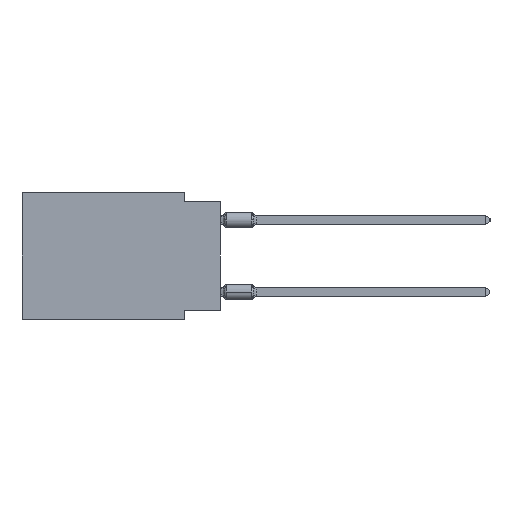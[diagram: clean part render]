
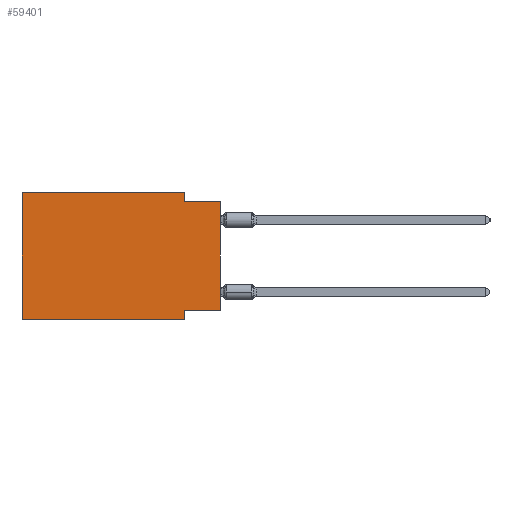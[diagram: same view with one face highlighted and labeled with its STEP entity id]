
A CAD part, left-side view. The second image highlights one B-rep face of the part: STEP entity #59401.
In plain terms, the highlighted planar face has unit normal (-1, 0, 0).
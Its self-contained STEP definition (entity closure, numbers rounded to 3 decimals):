
#155 = ORIENTED_EDGE ( 'NONE', *, *, #10946, .F. ) ;
#439 = DIRECTION ( 'NONE',  ( 0., -1., 0. ) ) ;
#2168 = DIRECTION ( 'NONE',  ( 0., 0., -1. ) ) ;
#2328 = CARTESIAN_POINT ( 'NONE',  ( 0., 13.97, -8.89 ) ) ;
#3798 = CARTESIAN_POINT ( 'NONE',  ( 0., 13.97, 0. ) ) ;
#4429 = DIRECTION ( 'NONE',  ( 0., 0., 1. ) ) ;
#4997 = VERTEX_POINT ( 'NONE', #58308 ) ;
#5055 = LINE ( 'NONE', #38365, #21850 ) ;
#5724 = VERTEX_POINT ( 'NONE', #56648 ) ;
#5874 = VECTOR ( 'NONE', #4429, 1000. ) ;
#6371 = CARTESIAN_POINT ( 'NONE',  ( 0., 0., -8.255 ) ) ;
#6458 = CARTESIAN_POINT ( 'NONE',  ( 0., 2.54, -8.89 ) ) ;
#7206 = VECTOR ( 'NONE', #55084, 1000. ) ;
#7301 = EDGE_CURVE ( 'NONE', #29168, #5724, #11497, .T. ) ;
#7315 = DIRECTION ( 'NONE',  ( 0., -1., 0. ) ) ;
#7899 = CARTESIAN_POINT ( 'NONE',  ( 0., 13.97, -8.89 ) ) ;
#8772 = VECTOR ( 'NONE', #9149, 1000. ) ;
#8821 = LINE ( 'NONE', #27630, #56164 ) ;
#9149 = DIRECTION ( 'NONE',  ( 0., 1., 0. ) ) ;
#9258 = VERTEX_POINT ( 'NONE', #46774 ) ;
#9321 = EDGE_CURVE ( 'NONE', #30063, #37108, #8821, .T. ) ;
#9517 = ORIENTED_EDGE ( 'NONE', *, *, #58188, .F. ) ;
#9600 = EDGE_LOOP ( 'NONE', ( #11555, #54944, #9517, #24430, #43706, #43105, #25051, #155 ) ) ;
#9776 = VECTOR ( 'NONE', #7315, 1000. ) ;
#10946 = EDGE_CURVE ( 'NONE', #29168, #9258, #13748, .T. ) ;
#11497 = LINE ( 'NONE', #24757, #60347 ) ;
#11555 = ORIENTED_EDGE ( 'NONE', *, *, #7301, .T. ) ;
#13257 = VERTEX_POINT ( 'NONE', #2328 ) ;
#13748 = LINE ( 'NONE', #51395, #8772 ) ;
#14059 = AXIS2_PLACEMENT_3D ( 'NONE', #25601, #31442, #2168 ) ;
#16603 = DIRECTION ( 'NONE',  ( 0., 0., -1. ) ) ;
#20598 = EDGE_CURVE ( 'NONE', #13257, #30063, #37748, .T. ) ;
#21850 = VECTOR ( 'NONE', #439, 1000. ) ;
#24430 = ORIENTED_EDGE ( 'NONE', *, *, #9321, .F. ) ;
#24757 = CARTESIAN_POINT ( 'NONE',  ( 0., 0., 0. ) ) ;
#25051 = ORIENTED_EDGE ( 'NONE', *, *, #44310, .F. ) ;
#25488 = CARTESIAN_POINT ( 'NONE',  ( 0., 2.54, 0. ) ) ;
#25601 = CARTESIAN_POINT ( 'NONE',  ( 0., 13.97, 0. ) ) ;
#26821 = FACE_OUTER_BOUND ( 'NONE', #9600, .T. ) ;
#26970 = VECTOR ( 'NONE', #16603, 1000. ) ;
#27630 = CARTESIAN_POINT ( 'NONE',  ( 0., 13.97, 0. ) ) ;
#29168 = VERTEX_POINT ( 'NONE', #6371 ) ;
#30063 = VERTEX_POINT ( 'NONE', #37222 ) ;
#30536 = PLANE ( 'NONE',  #14059 ) ;
#31442 = DIRECTION ( 'NONE',  ( 1., 0., 0. ) ) ;
#35159 = CARTESIAN_POINT ( 'NONE',  ( 0., 2.54, -0.635 ) ) ;
#36289 = CARTESIAN_POINT ( 'NONE',  ( 0., 2.54, 0. ) ) ;
#37108 = VERTEX_POINT ( 'NONE', #25488 ) ;
#37222 = CARTESIAN_POINT ( 'NONE',  ( 0., 13.97, 0. ) ) ;
#37748 = LINE ( 'NONE', #3798, #5874 ) ;
#38365 = CARTESIAN_POINT ( 'NONE',  ( 0., 0., -0.635 ) ) ;
#40601 = EDGE_CURVE ( 'NONE', #49997, #5724, #5055, .T. ) ;
#40626 = LINE ( 'NONE', #7899, #9776 ) ;
#43105 = ORIENTED_EDGE ( 'NONE', *, *, #46765, .T. ) ;
#43706 = ORIENTED_EDGE ( 'NONE', *, *, #20598, .F. ) ;
#44310 = EDGE_CURVE ( 'NONE', #9258, #4997, #58858, .T. ) ;
#46457 = DIRECTION ( 'NONE',  ( 0., -1., 0. ) ) ;
#46765 = EDGE_CURVE ( 'NONE', #13257, #4997, #40626, .T. ) ;
#46774 = CARTESIAN_POINT ( 'NONE',  ( 0., 2.54, -8.255 ) ) ;
#49436 = DIRECTION ( 'NONE',  ( 0., 0., 1. ) ) ;
#49997 = VERTEX_POINT ( 'NONE', #35159 ) ;
#51395 = CARTESIAN_POINT ( 'NONE',  ( 0., 0., -8.255 ) ) ;
#54944 = ORIENTED_EDGE ( 'NONE', *, *, #40601, .F. ) ;
#55084 = DIRECTION ( 'NONE',  ( 0., 0., -1. ) ) ;
#56164 = VECTOR ( 'NONE', #46457, 1000. ) ;
#56648 = CARTESIAN_POINT ( 'NONE',  ( 0., 0., -0.635 ) ) ;
#58188 = EDGE_CURVE ( 'NONE', #37108, #49997, #59732, .T. ) ;
#58308 = CARTESIAN_POINT ( 'NONE',  ( 0., 2.54, -8.89 ) ) ;
#58858 = LINE ( 'NONE', #6458, #26970 ) ;
#59401 = ADVANCED_FACE ( 'NONE', ( #26821 ), #30536, .F. ) ;
#59732 = LINE ( 'NONE', #36289, #7206 ) ;
#60347 = VECTOR ( 'NONE', #49436, 1000. ) ;
